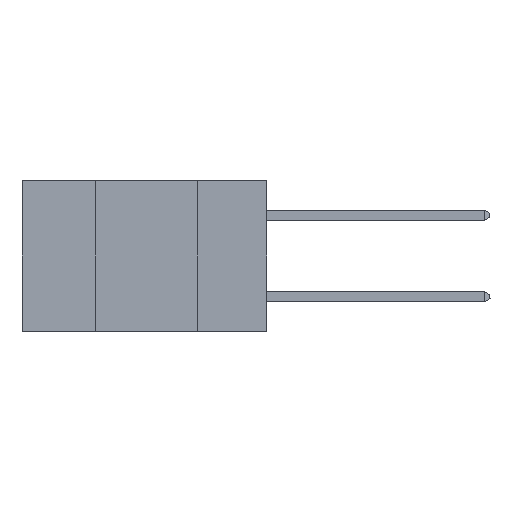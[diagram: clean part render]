
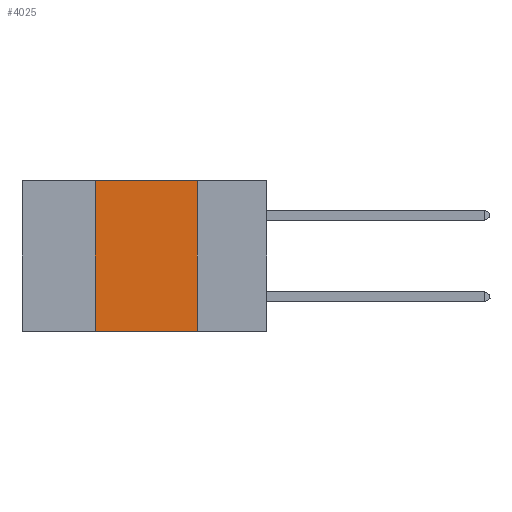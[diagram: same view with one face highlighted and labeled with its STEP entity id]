
A CAD part, left-side view. The second image highlights one B-rep face of the part: STEP entity #4025.
In plain terms, the highlighted planar face has unit normal (-1, 0, 0).
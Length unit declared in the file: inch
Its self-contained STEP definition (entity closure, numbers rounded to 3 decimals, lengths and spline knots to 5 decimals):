
#480 = VECTOR ( 'NONE', #11898, 39.37008 ) ;
#952 = VECTOR ( 'NONE', #22737, 39.37008 ) ;
#1833 = ORIENTED_EDGE ( 'NONE', *, *, #19949, .F. ) ;
#4025 = ADVANCED_FACE ( 'NONE', ( #25485 ), #30121, .F. ) ;
#4184 = DIRECTION ( 'NONE',  ( 0., 0., 1. ) ) ;
#4225 = CARTESIAN_POINT ( 'NONE',  ( 0., 0.42, 0. ) ) ;
#5786 = CARTESIAN_POINT ( 'NONE',  ( 0., 0.42, 0. ) ) ;
#5799 = VERTEX_POINT ( 'NONE', #8053 ) ;
#6506 = LINE ( 'NONE', #20142, #952 ) ;
#6604 = LINE ( 'NONE', #21250, #16330 ) ;
#7008 = VECTOR ( 'NONE', #4184, 39.37008 ) ;
#7622 = VERTEX_POINT ( 'NONE', #26227 ) ;
#8053 = CARTESIAN_POINT ( 'NONE',  ( 0., 0.17, -0.37 ) ) ;
#9448 = CARTESIAN_POINT ( 'NONE',  ( 0., 0.42, -0.37 ) ) ;
#10846 = LINE ( 'NONE', #5786, #7008 ) ;
#11668 = CARTESIAN_POINT ( 'NONE',  ( 0., 0.6, 0. ) ) ;
#11898 = DIRECTION ( 'NONE',  ( 0., -1., 0. ) ) ;
#14358 = EDGE_CURVE ( 'NONE', #22507, #7622, #26763, .T. ) ;
#16330 = VECTOR ( 'NONE', #18971, 39.37008 ) ;
#17763 = DIRECTION ( 'NONE',  ( 1., 0., 0. ) ) ;
#17965 = DIRECTION ( 'NONE',  ( 0., 0., -1. ) ) ;
#18971 = DIRECTION ( 'NONE',  ( 0., 0., -1. ) ) ;
#19949 = EDGE_CURVE ( 'NONE', #7622, #5799, #6604, .T. ) ;
#20142 = CARTESIAN_POINT ( 'NONE',  ( 0., 0.6, -0.37 ) ) ;
#20715 = EDGE_CURVE ( 'NONE', #23766, #22507, #10846, .T. ) ;
#21250 = CARTESIAN_POINT ( 'NONE',  ( 0., 0.17, 0. ) ) ;
#22507 = VERTEX_POINT ( 'NONE', #4225 ) ;
#22737 = DIRECTION ( 'NONE',  ( 0., -1., 0. ) ) ;
#23437 = AXIS2_PLACEMENT_3D ( 'NONE', #27716, #17763, #17965 ) ;
#23766 = VERTEX_POINT ( 'NONE', #9448 ) ;
#24129 = EDGE_CURVE ( 'NONE', #23766, #5799, #6506, .T. ) ;
#24712 = ORIENTED_EDGE ( 'NONE', *, *, #14358, .F. ) ;
#25485 = FACE_OUTER_BOUND ( 'NONE', #32317, .T. ) ;
#26227 = CARTESIAN_POINT ( 'NONE',  ( 0., 0.17, 0. ) ) ;
#26763 = LINE ( 'NONE', #11668, #480 ) ;
#27716 = CARTESIAN_POINT ( 'NONE',  ( 0., 0.6, 0. ) ) ;
#27793 = ORIENTED_EDGE ( 'NONE', *, *, #24129, .T. ) ;
#30121 = PLANE ( 'NONE',  #23437 ) ;
#30433 = ORIENTED_EDGE ( 'NONE', *, *, #20715, .F. ) ;
#32317 = EDGE_LOOP ( 'NONE', ( #1833, #24712, #30433, #27793 ) ) ;
